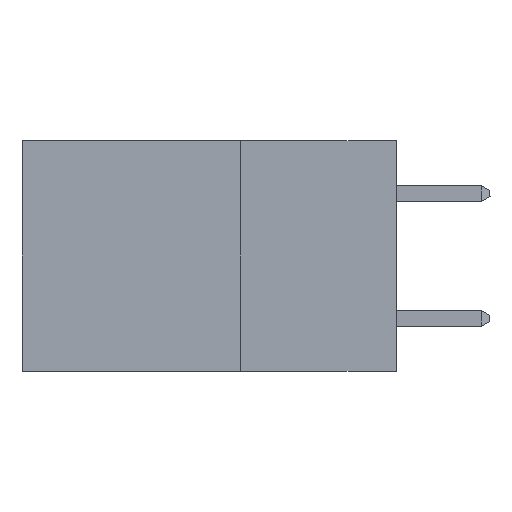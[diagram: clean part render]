
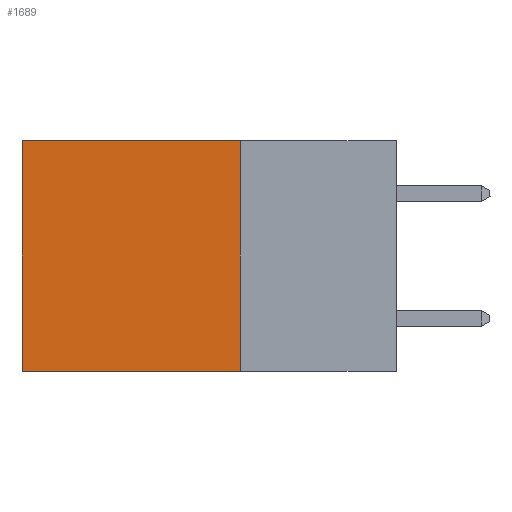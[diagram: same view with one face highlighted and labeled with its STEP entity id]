
A CAD part, left-side view. The second image highlights one B-rep face of the part: STEP entity #1689.
In plain terms, the highlighted planar face has unit normal (-1, 0, 0).
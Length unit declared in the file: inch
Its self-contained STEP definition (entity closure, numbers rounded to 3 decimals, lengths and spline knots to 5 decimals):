
#13 = VECTOR ( 'NONE', #8126, 39.37008 ) ;
#518 = ORIENTED_EDGE ( 'NONE', *, *, #3445, .F. ) ;
#1184 = LINE ( 'NONE', #3804, #13 ) ;
#1234 = DIRECTION ( 'NONE',  ( 1., 0., 0. ) ) ;
#1689 = ADVANCED_FACE ( 'NONE', ( #7590 ), #4450, .F. ) ;
#1726 = ORIENTED_EDGE ( 'NONE', *, *, #5315, .T. ) ;
#2272 = EDGE_CURVE ( 'NONE', #8785, #11545, #8505, .T. ) ;
#2340 = VECTOR ( 'NONE', #7461, 39.37008 ) ;
#3445 = EDGE_CURVE ( 'NONE', #7207, #10991, #4160, .T. ) ;
#3804 = CARTESIAN_POINT ( 'NONE',  ( 0.298, 0.25, -0.37 ) ) ;
#3848 = ORIENTED_EDGE ( 'NONE', *, *, #2272, .T. ) ;
#3923 = LINE ( 'NONE', #7768, #11267 ) ;
#4160 = LINE ( 'NONE', #4548, #9157 ) ;
#4331 = EDGE_LOOP ( 'NONE', ( #3848, #8531, #518, #1726 ) ) ;
#4450 = PLANE ( 'NONE',  #9391 ) ;
#4548 = CARTESIAN_POINT ( 'NONE',  ( 0.298, 0.25, 0. ) ) ;
#5315 = EDGE_CURVE ( 'NONE', #7207, #8785, #3923, .T. ) ;
#5965 = CARTESIAN_POINT ( 'NONE',  ( 0.298, 0.6, -0.37 ) ) ;
#7207 = VERTEX_POINT ( 'NONE', #9296 ) ;
#7461 = DIRECTION ( 'NONE',  ( 0., 0., -1. ) ) ;
#7590 = FACE_OUTER_BOUND ( 'NONE', #4331, .T. ) ;
#7690 = DIRECTION ( 'NONE',  ( 0., 0., -1. ) ) ;
#7768 = CARTESIAN_POINT ( 'NONE',  ( 0.298, 0.25, 0. ) ) ;
#8088 = DIRECTION ( 'NONE',  ( 0., 1., 0. ) ) ;
#8126 = DIRECTION ( 'NONE',  ( 0., 1., 0. ) ) ;
#8505 = LINE ( 'NONE', #10680, #2340 ) ;
#8531 = ORIENTED_EDGE ( 'NONE', *, *, #11563, .F. ) ;
#8785 = VERTEX_POINT ( 'NONE', #11182 ) ;
#9157 = VECTOR ( 'NONE', #7690, 39.37008 ) ;
#9296 = CARTESIAN_POINT ( 'NONE',  ( 0.298, 0.25, 0. ) ) ;
#9391 = AXIS2_PLACEMENT_3D ( 'NONE', #10978, #1234, #13083 ) ;
#10459 = CARTESIAN_POINT ( 'NONE',  ( 0.298, 0.25, -0.37 ) ) ;
#10680 = CARTESIAN_POINT ( 'NONE',  ( 0.298, 0.6, 0. ) ) ;
#10978 = CARTESIAN_POINT ( 'NONE',  ( 0.298, 0.25, 0. ) ) ;
#10991 = VERTEX_POINT ( 'NONE', #10459 ) ;
#11182 = CARTESIAN_POINT ( 'NONE',  ( 0.298, 0.6, 0. ) ) ;
#11267 = VECTOR ( 'NONE', #8088, 39.37008 ) ;
#11545 = VERTEX_POINT ( 'NONE', #5965 ) ;
#11563 = EDGE_CURVE ( 'NONE', #10991, #11545, #1184, .T. ) ;
#13083 = DIRECTION ( 'NONE',  ( 0., 0., -1. ) ) ;
